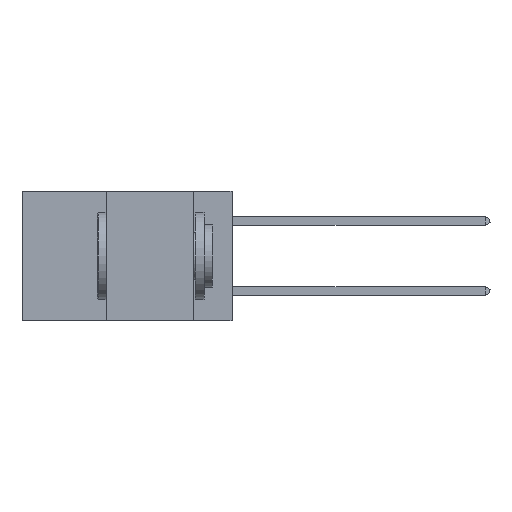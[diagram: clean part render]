
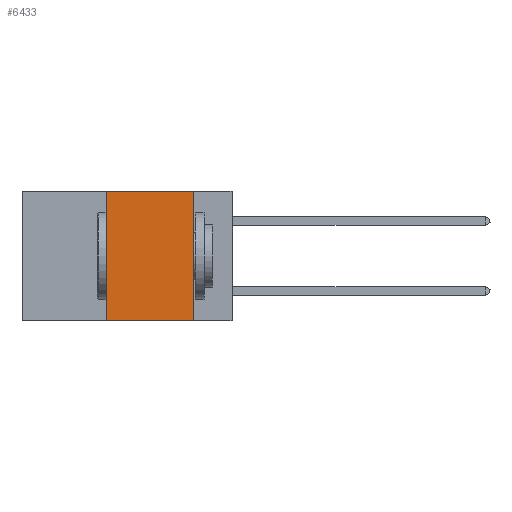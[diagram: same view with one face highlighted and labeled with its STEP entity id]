
A CAD part, left-side view. The second image highlights one B-rep face of the part: STEP entity #6433.
In plain terms, the highlighted planar face has unit normal (-1, 0, 0).
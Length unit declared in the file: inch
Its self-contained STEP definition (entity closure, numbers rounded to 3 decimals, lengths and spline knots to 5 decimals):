
#1530 = EDGE_CURVE ( 'NONE', #15414, #3971, #12655, .T. ) ;
#2204 = LINE ( 'NONE', #4839, #12940 ) ;
#2736 = VERTEX_POINT ( 'NONE', #7727 ) ;
#2915 = EDGE_CURVE ( 'NONE', #15414, #2736, #2204, .T. ) ;
#3790 = VECTOR ( 'NONE', #23434, 39.37008 ) ;
#3971 = VERTEX_POINT ( 'NONE', #7854 ) ;
#4839 = CARTESIAN_POINT ( 'NONE',  ( 0., 0.6, -0.37 ) ) ;
#4887 = ORIENTED_EDGE ( 'NONE', *, *, #1530, .F. ) ;
#4960 = DIRECTION ( 'NONE',  ( 0., -1., 0. ) ) ;
#5993 = VECTOR ( 'NONE', #10068, 39.37008 ) ;
#6433 = ADVANCED_FACE ( 'NONE', ( #19450 ), #11141, .F. ) ;
#7727 = CARTESIAN_POINT ( 'NONE',  ( 0., 0.11, -0.37 ) ) ;
#7854 = CARTESIAN_POINT ( 'NONE',  ( 0., 0.36, 0. ) ) ;
#9063 = CARTESIAN_POINT ( 'NONE',  ( 0., 0.36, -0.37 ) ) ;
#10068 = DIRECTION ( 'NONE',  ( 0., -1., 0. ) ) ;
#11141 = PLANE ( 'NONE',  #25661 ) ;
#12655 = LINE ( 'NONE', #15351, #17798 ) ;
#12940 = VECTOR ( 'NONE', #4960, 39.37008 ) ;
#13123 = DIRECTION ( 'NONE',  ( 0., 0., -1. ) ) ;
#13386 = ORIENTED_EDGE ( 'NONE', *, *, #19477, .F. ) ;
#15351 = CARTESIAN_POINT ( 'NONE',  ( 0., 0.36, 0. ) ) ;
#15414 = VERTEX_POINT ( 'NONE', #9063 ) ;
#15827 = ORIENTED_EDGE ( 'NONE', *, *, #24583, .F. ) ;
#16664 = ORIENTED_EDGE ( 'NONE', *, *, #2915, .T. ) ;
#16904 = CARTESIAN_POINT ( 'NONE',  ( 0., 0.6, 0. ) ) ;
#17798 = VECTOR ( 'NONE', #22647, 39.37008 ) ;
#19125 = CARTESIAN_POINT ( 'NONE',  ( 0., 0.11, 0. ) ) ;
#19450 = FACE_OUTER_BOUND ( 'NONE', #24109, .T. ) ;
#19477 = EDGE_CURVE ( 'NONE', #3971, #21811, #20990, .T. ) ;
#19520 = LINE ( 'NONE', #23809, #3790 ) ;
#20990 = LINE ( 'NONE', #21722, #5993 ) ;
#21722 = CARTESIAN_POINT ( 'NONE',  ( 0., 0.6, 0. ) ) ;
#21811 = VERTEX_POINT ( 'NONE', #19125 ) ;
#22647 = DIRECTION ( 'NONE',  ( 0., 0., 1. ) ) ;
#23434 = DIRECTION ( 'NONE',  ( 0., 0., -1. ) ) ;
#23809 = CARTESIAN_POINT ( 'NONE',  ( 0., 0.11, 0. ) ) ;
#24109 = EDGE_LOOP ( 'NONE', ( #15827, #13386, #4887, #16664 ) ) ;
#24583 = EDGE_CURVE ( 'NONE', #21811, #2736, #19520, .T. ) ;
#24755 = DIRECTION ( 'NONE',  ( 1., 0., 0. ) ) ;
#25661 = AXIS2_PLACEMENT_3D ( 'NONE', #16904, #24755, #13123 ) ;
